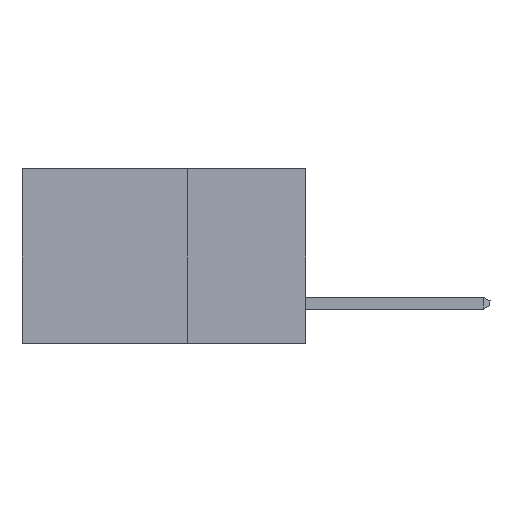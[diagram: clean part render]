
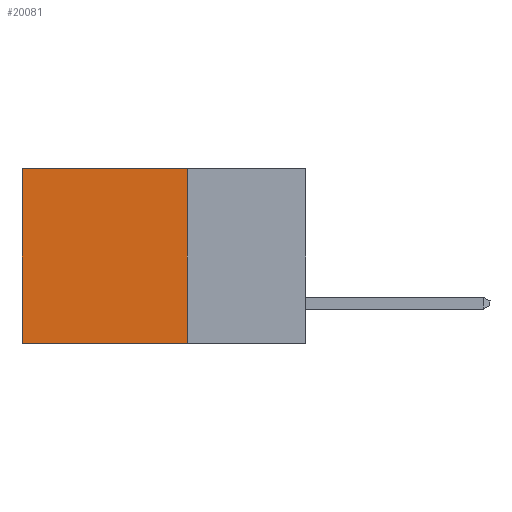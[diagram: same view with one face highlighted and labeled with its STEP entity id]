
A CAD part, left-side view. The second image highlights one B-rep face of the part: STEP entity #20081.
In plain terms, the highlighted planar face has unit normal (-1, 0, 0).
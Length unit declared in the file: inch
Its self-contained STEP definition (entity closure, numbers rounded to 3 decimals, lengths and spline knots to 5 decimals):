
#58 = VECTOR ( 'NONE', #4932, 39.37008 ) ;
#277 = ORIENTED_EDGE ( 'NONE', *, *, #9868, .F. ) ;
#286 = PLANE ( 'NONE',  #8369 ) ;
#1816 = ORIENTED_EDGE ( 'NONE', *, *, #21060, .T. ) ;
#2200 = DIRECTION ( 'NONE',  ( 0., 0., -1. ) ) ;
#2454 = VERTEX_POINT ( 'NONE', #19173 ) ;
#3411 = CARTESIAN_POINT ( 'NONE',  ( 0.2615, 0.25, -0.37 ) ) ;
#4932 = DIRECTION ( 'NONE',  ( 0., 1., 0. ) ) ;
#6173 = DIRECTION ( 'NONE',  ( 0., 0., -1. ) ) ;
#6277 = EDGE_CURVE ( 'NONE', #13044, #2454, #15540, .T. ) ;
#6687 = CARTESIAN_POINT ( 'NONE',  ( 0.2615, 0.25, -0.37 ) ) ;
#7299 = ORIENTED_EDGE ( 'NONE', *, *, #6277, .F. ) ;
#8369 = AXIS2_PLACEMENT_3D ( 'NONE', #11643, #13468, #2200 ) ;
#9868 = EDGE_CURVE ( 'NONE', #22033, #13044, #15814, .T. ) ;
#11074 = VECTOR ( 'NONE', #6173, 39.37008 ) ;
#11274 = CARTESIAN_POINT ( 'NONE',  ( 0.2615, 0.25, 0. ) ) ;
#11528 = VERTEX_POINT ( 'NONE', #14560 ) ;
#11643 = CARTESIAN_POINT ( 'NONE',  ( 0.2615, 0.25, -0.37 ) ) ;
#13044 = VERTEX_POINT ( 'NONE', #3411 ) ;
#13178 = EDGE_CURVE ( 'NONE', #11528, #2454, #17435, .T. ) ;
#13468 = DIRECTION ( 'NONE',  ( 1., 0., 0. ) ) ;
#14560 = CARTESIAN_POINT ( 'NONE',  ( 0.2615, 0.6, 0. ) ) ;
#14597 = ORIENTED_EDGE ( 'NONE', *, *, #13178, .T. ) ;
#15540 = LINE ( 'NONE', #18470, #58 ) ;
#15594 = EDGE_LOOP ( 'NONE', ( #14597, #7299, #277, #1816 ) ) ;
#15814 = LINE ( 'NONE', #6687, #11074 ) ;
#17435 = LINE ( 'NONE', #23203, #22436 ) ;
#18470 = CARTESIAN_POINT ( 'NONE',  ( 0.2615, 0.25, -0.37 ) ) ;
#19173 = CARTESIAN_POINT ( 'NONE',  ( 0.2615, 0.6, -0.37 ) ) ;
#20081 = ADVANCED_FACE ( 'NONE', ( #20366 ), #286, .F. ) ;
#20366 = FACE_OUTER_BOUND ( 'NONE', #15594, .T. ) ;
#21060 = EDGE_CURVE ( 'NONE', #22033, #11528, #21103, .T. ) ;
#21103 = LINE ( 'NONE', #11274, #22135 ) ;
#22033 = VERTEX_POINT ( 'NONE', #22723 ) ;
#22135 = VECTOR ( 'NONE', #23245, 39.37008 ) ;
#22436 = VECTOR ( 'NONE', #23115, 39.37008 ) ;
#22723 = CARTESIAN_POINT ( 'NONE',  ( 0.2615, 0.25, 0. ) ) ;
#23115 = DIRECTION ( 'NONE',  ( 0., 0., -1. ) ) ;
#23203 = CARTESIAN_POINT ( 'NONE',  ( 0.2615, 0.6, -0.37 ) ) ;
#23245 = DIRECTION ( 'NONE',  ( 0., 1., 0. ) ) ;
